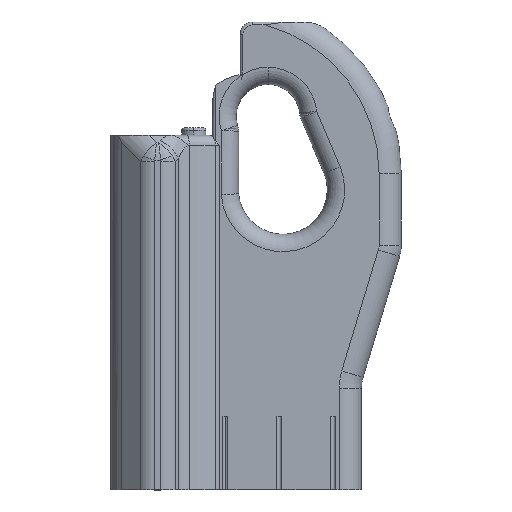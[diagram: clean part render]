
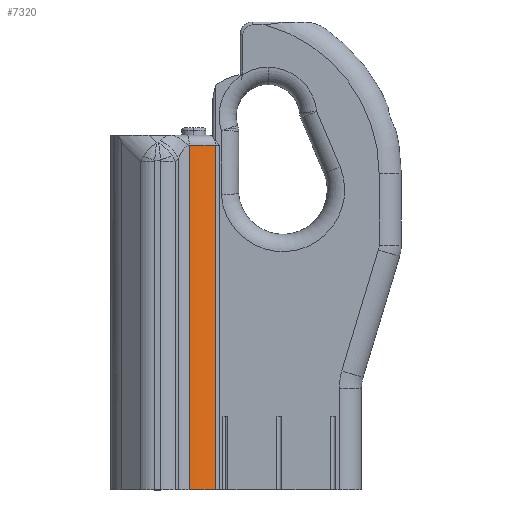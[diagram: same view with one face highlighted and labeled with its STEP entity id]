
A CAD part, left-side view. The second image highlights one B-rep face of the part: STEP entity #7320.
In plain terms, the highlighted cylindrical face has radius 35 mm (diameter 70 mm), a partial arc.
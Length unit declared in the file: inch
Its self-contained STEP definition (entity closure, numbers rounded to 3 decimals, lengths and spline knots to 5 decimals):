
#86 = AXIS2_PLACEMENT_3D ( 'NONE', #1252, #580, #4972 ) ;
#226 = CARTESIAN_POINT ( 'NONE',  ( 4.26914, 6.70065, 8.61076 ) ) ;
#526 = ORIENTED_EDGE ( 'NONE', *, *, #5566, .T. ) ;
#580 = DIRECTION ( 'NONE',  ( 0., 0., 1. ) ) ;
#800 = FACE_OUTER_BOUND ( 'NONE', #3141, .T. ) ;
#984 = CIRCLE ( 'NONE', #4488, 1.37795 ) ;
#1252 = CARTESIAN_POINT ( 'NONE',  ( 5.62236, 6.96053, 12.08462 ) ) ;
#1299 = EDGE_CURVE ( 'NONE', #5662, #3785, #984, .T. ) ;
#2122 = CARTESIAN_POINT ( 'NONE',  ( 4.26914, 6.70065, 1.57196 ) ) ;
#2516 = CARTESIAN_POINT ( 'NONE',  ( 4.26914, 6.70065, 12.08462 ) ) ;
#2878 = VECTOR ( 'NONE', #7776, 39.37008 ) ;
#3141 = EDGE_LOOP ( 'NONE', ( #7539, #526, #5867, #3349 ) ) ;
#3297 = LINE ( 'NONE', #2516, #8034 ) ;
#3349 = ORIENTED_EDGE ( 'NONE', *, *, #1299, .F. ) ;
#3630 = CARTESIAN_POINT ( 'NONE',  ( 4.4973, 6.16493, 1.57196 ) ) ;
#3785 = VERTEX_POINT ( 'NONE', #2122 ) ;
#3792 = DIRECTION ( 'NONE',  ( -1., 0., 0. ) ) ;
#3798 = DIRECTION ( 'NONE',  ( 0., 0., -1. ) ) ;
#3807 = CARTESIAN_POINT ( 'NONE',  ( 4.4973, 6.16493, 8.61076 ) ) ;
#3809 = CARTESIAN_POINT ( 'NONE',  ( 5.62236, 6.96053, 1.57196 ) ) ;
#4488 = AXIS2_PLACEMENT_3D ( 'NONE', #3809, #3798, #3792 ) ;
#4523 = LINE ( 'NONE', #7369, #2878 ) ;
#4675 = DIRECTION ( 'NONE',  ( 1., 0., 0. ) ) ;
#4712 = DIRECTION ( 'NONE',  ( 0., 0., -1. ) ) ;
#4719 = CARTESIAN_POINT ( 'NONE',  ( 5.62236, 6.96053, 8.61076 ) ) ;
#4747 = CYLINDRICAL_SURFACE ( 'NONE', #86, 1.37795 ) ;
#4972 = DIRECTION ( 'NONE',  ( 1., 0., 0. ) ) ;
#5379 = EDGE_CURVE ( 'NONE', #6272, #5662, #4523, .T. ) ;
#5566 = EDGE_CURVE ( 'NONE', #6272, #7738, #5825, .T. ) ;
#5662 = VERTEX_POINT ( 'NONE', #3630 ) ;
#5825 = CIRCLE ( 'NONE', #6268, 1.37795 ) ;
#5867 = ORIENTED_EDGE ( 'NONE', *, *, #7321, .T. ) ;
#6268 = AXIS2_PLACEMENT_3D ( 'NONE', #4719, #4712, #4675 ) ;
#6272 = VERTEX_POINT ( 'NONE', #3807 ) ;
#6851 = DIRECTION ( 'NONE',  ( 0., 0., -1. ) ) ;
#7320 = ADVANCED_FACE ( 'NONE', ( #800 ), #4747, .T. ) ;
#7321 = EDGE_CURVE ( 'NONE', #7738, #3785, #3297, .T. ) ;
#7369 = CARTESIAN_POINT ( 'NONE',  ( 4.4973, 6.16493, 12.08462 ) ) ;
#7539 = ORIENTED_EDGE ( 'NONE', *, *, #5379, .F. ) ;
#7738 = VERTEX_POINT ( 'NONE', #226 ) ;
#7776 = DIRECTION ( 'NONE',  ( 0., 0., -1. ) ) ;
#8034 = VECTOR ( 'NONE', #6851, 39.37008 ) ;
